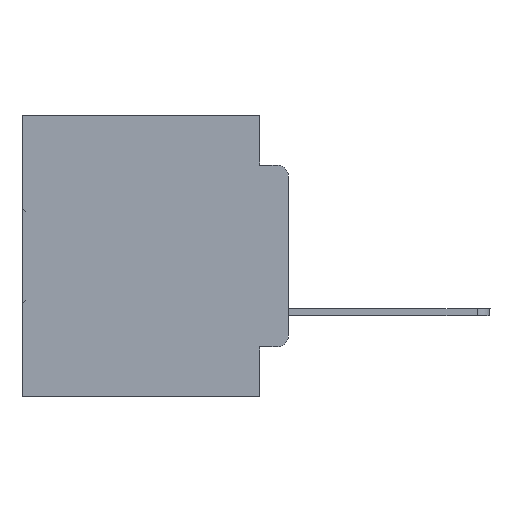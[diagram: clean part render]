
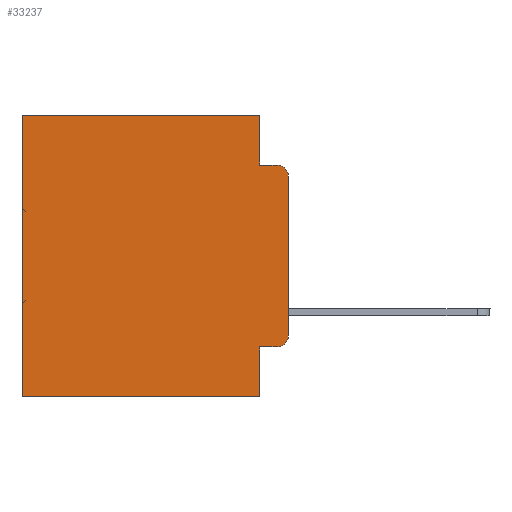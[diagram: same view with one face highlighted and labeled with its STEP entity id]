
A CAD part, left-side view. The second image highlights one B-rep face of the part: STEP entity #33237.
In plain terms, the highlighted planar face has unit normal (-1, 0, 0).
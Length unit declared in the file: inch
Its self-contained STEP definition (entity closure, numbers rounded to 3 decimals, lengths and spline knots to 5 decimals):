
#698 = VERTEX_POINT ( 'NONE', #2674 ) ;
#890 = DIRECTION ( 'NONE',  ( 0., -1., 0. ) ) ;
#956 = VECTOR ( 'NONE', #890, 39.37008 ) ;
#1669 = ORIENTED_EDGE ( 'NONE', *, *, #9277, .F. ) ;
#1877 = EDGE_CURVE ( 'NONE', #14995, #11469, #19011, .T. ) ;
#2496 = EDGE_CURVE ( 'NONE', #28444, #5995, #13321, .T. ) ;
#2600 = DIRECTION ( 'NONE',  ( 0., 0., -1. ) ) ;
#2674 = CARTESIAN_POINT ( 'NONE',  ( 0.298, 0.051, -0.4115 ) ) ;
#3124 = CARTESIAN_POINT ( 'NONE',  ( 0.298, 0., -0.5 ) ) ;
#3169 = VECTOR ( 'NONE', #31821, 39.37008 ) ;
#3574 = DIRECTION ( 'NONE',  ( 0., 0., -1. ) ) ;
#4776 = VERTEX_POINT ( 'NONE', #7551 ) ;
#4981 = EDGE_CURVE ( 'NONE', #11469, #14128, #11250, .T. ) ;
#5056 = DIRECTION ( 'NONE',  ( 0., -1., 0. ) ) ;
#5474 = AXIS2_PLACEMENT_3D ( 'NONE', #13276, #7871, #2600 ) ;
#5950 = ORIENTED_EDGE ( 'NONE', *, *, #8215, .F. ) ;
#5995 = VERTEX_POINT ( 'NONE', #12332 ) ;
#6148 = DIRECTION ( 'NONE',  ( 0., 0., -1. ) ) ;
#6238 = ORIENTED_EDGE ( 'NONE', *, *, #18979, .T. ) ;
#6565 = ORIENTED_EDGE ( 'NONE', *, *, #31816, .T. ) ;
#7160 = VECTOR ( 'NONE', #30382, 39.37008 ) ;
#7551 = CARTESIAN_POINT ( 'NONE',  ( 0.298, 0.051, -0.5 ) ) ;
#7613 = LINE ( 'NONE', #14881, #12171 ) ;
#7871 = DIRECTION ( 'NONE',  ( -1., 0., 0. ) ) ;
#8215 = EDGE_CURVE ( 'NONE', #4776, #5995, #26485, .T. ) ;
#8626 = EDGE_CURVE ( 'NONE', #698, #4776, #14776, .T. ) ;
#8894 = CIRCLE ( 'NONE', #21371, 0.02 ) ;
#9277 = EDGE_CURVE ( 'NONE', #14125, #26061, #24026, .T. ) ;
#9578 = DIRECTION ( 'NONE',  ( 1., 0., 0. ) ) ;
#9836 = VECTOR ( 'NONE', #18410, 39.37008 ) ;
#10016 = ORIENTED_EDGE ( 'NONE', *, *, #4981, .F. ) ;
#10112 = DIRECTION ( 'NONE',  ( 0., 0., -1. ) ) ;
#11085 = EDGE_LOOP ( 'NONE', ( #1669, #31221, #10016, #28628, #6238, #25235, #5950, #24342, #6565, #11280 ) ) ;
#11250 = LINE ( 'NONE', #28867, #956 ) ;
#11280 = ORIENTED_EDGE ( 'NONE', *, *, #31130, .T. ) ;
#11434 = CARTESIAN_POINT ( 'NONE',  ( 0.298, 0.473, 0. ) ) ;
#11469 = VERTEX_POINT ( 'NONE', #19720 ) ;
#12171 = VECTOR ( 'NONE', #5056, 39.37008 ) ;
#12332 = CARTESIAN_POINT ( 'NONE',  ( 0.298, 0.473, -0.5 ) ) ;
#12906 = CARTESIAN_POINT ( 'NONE',  ( 0.298, 0.02, -0.0885 ) ) ;
#13276 = CARTESIAN_POINT ( 'NONE',  ( 0.298, 0.02, -0.1085 ) ) ;
#13321 = LINE ( 'NONE', #11434, #9836 ) ;
#13696 = LINE ( 'NONE', #14365, #16457 ) ;
#14125 = VERTEX_POINT ( 'NONE', #17979 ) ;
#14128 = VERTEX_POINT ( 'NONE', #12906 ) ;
#14365 = CARTESIAN_POINT ( 'NONE',  ( 0.298, 0., 0. ) ) ;
#14435 = CARTESIAN_POINT ( 'NONE',  ( 0.298, 0.051, 0. ) ) ;
#14648 = FACE_OUTER_BOUND ( 'NONE', #11085, .T. ) ;
#14723 = VECTOR ( 'NONE', #6148, 39.37008 ) ;
#14776 = LINE ( 'NONE', #22581, #7160 ) ;
#14881 = CARTESIAN_POINT ( 'NONE',  ( 0.298, 0.051, -0.4115 ) ) ;
#14995 = VERTEX_POINT ( 'NONE', #14435 ) ;
#15973 = AXIS2_PLACEMENT_3D ( 'NONE', #17541, #9578, #10112 ) ;
#16457 = VECTOR ( 'NONE', #29280, 39.37008 ) ;
#16617 = CARTESIAN_POINT ( 'NONE',  ( 0.298, 0.473, 0. ) ) ;
#17541 = CARTESIAN_POINT ( 'NONE',  ( 0.298, 0., 0. ) ) ;
#17979 = CARTESIAN_POINT ( 'NONE',  ( 0.298, 0., -0.1085 ) ) ;
#18410 = DIRECTION ( 'NONE',  ( 0., 0., -1. ) ) ;
#18519 = VECTOR ( 'NONE', #26649, 39.37008 ) ;
#18529 = CARTESIAN_POINT ( 'NONE',  ( 0.298, 0., -0.3915 ) ) ;
#18979 = EDGE_CURVE ( 'NONE', #14995, #28444, #13696, .T. ) ;
#19011 = LINE ( 'NONE', #29341, #14723 ) ;
#19457 = CARTESIAN_POINT ( 'NONE',  ( 0.298, 0., 0. ) ) ;
#19720 = CARTESIAN_POINT ( 'NONE',  ( 0.298, 0.051, -0.0885 ) ) ;
#20816 = CARTESIAN_POINT ( 'NONE',  ( 0.298, 0.02, -0.4115 ) ) ;
#21371 = AXIS2_PLACEMENT_3D ( 'NONE', #26787, #21567, #3574 ) ;
#21567 = DIRECTION ( 'NONE',  ( -1., 0., 0. ) ) ;
#22226 = CIRCLE ( 'NONE', #5474, 0.02 ) ;
#22581 = CARTESIAN_POINT ( 'NONE',  ( 0.298, 0.051, 0. ) ) ;
#24026 = LINE ( 'NONE', #19457, #3169 ) ;
#24342 = ORIENTED_EDGE ( 'NONE', *, *, #8626, .F. ) ;
#25235 = ORIENTED_EDGE ( 'NONE', *, *, #2496, .T. ) ;
#26061 = VERTEX_POINT ( 'NONE', #18529 ) ;
#26485 = LINE ( 'NONE', #3124, #18519 ) ;
#26649 = DIRECTION ( 'NONE',  ( 0., 1., 0. ) ) ;
#26787 = CARTESIAN_POINT ( 'NONE',  ( 0.298, 0.02, -0.3915 ) ) ;
#27517 = PLANE ( 'NONE',  #15973 ) ;
#27831 = EDGE_CURVE ( 'NONE', #14125, #14128, #22226, .T. ) ;
#28444 = VERTEX_POINT ( 'NONE', #16617 ) ;
#28628 = ORIENTED_EDGE ( 'NONE', *, *, #1877, .F. ) ;
#28867 = CARTESIAN_POINT ( 'NONE',  ( 0.298, 0.051, -0.0885 ) ) ;
#28976 = VERTEX_POINT ( 'NONE', #20816 ) ;
#29280 = DIRECTION ( 'NONE',  ( 0., 1., 0. ) ) ;
#29341 = CARTESIAN_POINT ( 'NONE',  ( 0.298, 0.051, 0. ) ) ;
#30382 = DIRECTION ( 'NONE',  ( 0., 0., -1. ) ) ;
#31130 = EDGE_CURVE ( 'NONE', #28976, #26061, #8894, .T. ) ;
#31221 = ORIENTED_EDGE ( 'NONE', *, *, #27831, .T. ) ;
#31816 = EDGE_CURVE ( 'NONE', #698, #28976, #7613, .T. ) ;
#31821 = DIRECTION ( 'NONE',  ( 0., 0., -1. ) ) ;
#33237 = ADVANCED_FACE ( 'NONE', ( #14648 ), #27517, .F. ) ;
